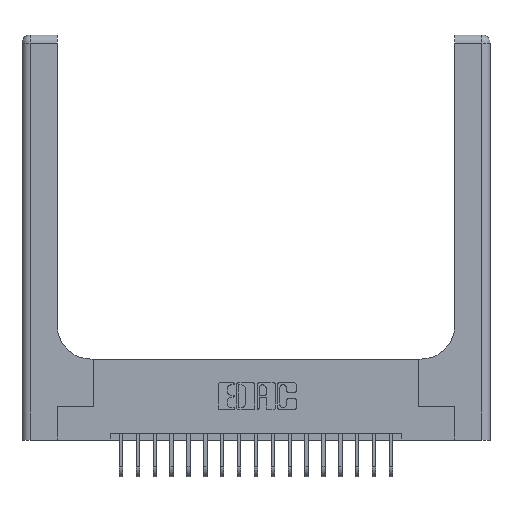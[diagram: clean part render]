
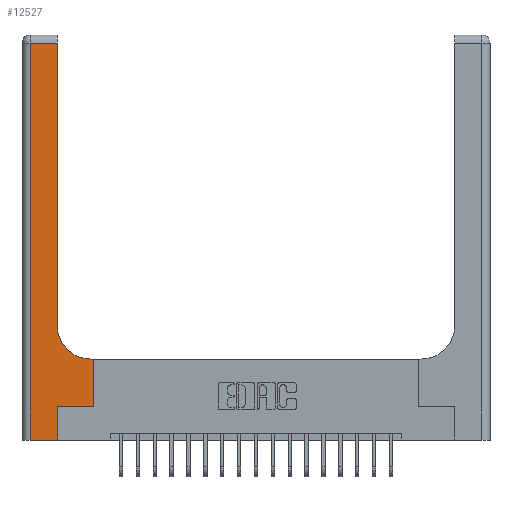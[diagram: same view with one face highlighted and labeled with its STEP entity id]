
A CAD part, top view. The second image highlights one B-rep face of the part: STEP entity #12527.
In plain terms, the highlighted planar face has unit normal (0, 0, 1).
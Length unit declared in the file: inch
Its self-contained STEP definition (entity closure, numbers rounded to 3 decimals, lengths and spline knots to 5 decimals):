
#15 = DIRECTION ( 'NONE',  ( 1., 0., 0. ) ) ;
#594 = VERTEX_POINT ( 'NONE', #11328 ) ;
#892 = CARTESIAN_POINT ( 'NONE',  ( 0.51, 0.85, 0.37 ) ) ;
#1143 = CARTESIAN_POINT ( 'NONE',  ( 0.265, 0., 0.37 ) ) ;
#1306 = VERTEX_POINT ( 'NONE', #5711 ) ;
#1952 = LINE ( 'NONE', #5058, #9387 ) ;
#2213 = LINE ( 'NONE', #4415, #17947 ) ;
#2278 = VECTOR ( 'NONE', #9556, 39.37008 ) ;
#2407 = DIRECTION ( 'NONE',  ( 1., 0., 0. ) ) ;
#2471 = VERTEX_POINT ( 'NONE', #10044 ) ;
#2762 = VERTEX_POINT ( 'NONE', #13661 ) ;
#2944 = VERTEX_POINT ( 'NONE', #16713 ) ;
#3166 = ORIENTED_EDGE ( 'NONE', *, *, #4257, .T. ) ;
#3633 = EDGE_CURVE ( 'NONE', #1306, #2944, #17541, .T. ) ;
#3646 = ORIENTED_EDGE ( 'NONE', *, *, #9079, .T. ) ;
#4257 = EDGE_CURVE ( 'NONE', #17319, #1306, #7355, .T. ) ;
#4364 = CIRCLE ( 'NONE', #14525, 0.25 ) ;
#4415 = CARTESIAN_POINT ( 'NONE',  ( 0.265, 0., 0.37 ) ) ;
#4584 = CARTESIAN_POINT ( 'NONE',  ( 0., 3., 0.37 ) ) ;
#4614 = LINE ( 'NONE', #6154, #12495 ) ;
#5058 = CARTESIAN_POINT ( 'NONE',  ( 0., 2.94, 0.37 ) ) ;
#5375 = FACE_OUTER_BOUND ( 'NONE', #8988, .T. ) ;
#5711 = CARTESIAN_POINT ( 'NONE',  ( 0.528, 0.25, 0.37 ) ) ;
#5756 = ORIENTED_EDGE ( 'NONE', *, *, #7714, .T. ) ;
#5978 = LINE ( 'NONE', #15850, #13363 ) ;
#6038 = DIRECTION ( 'NONE',  ( 0., -1., 0. ) ) ;
#6096 = DIRECTION ( 'NONE',  ( 0., 0., -1. ) ) ;
#6154 = CARTESIAN_POINT ( 'NONE',  ( 0.26, 3., 0.37 ) ) ;
#6441 = VECTOR ( 'NONE', #15, 39.37008 ) ;
#6572 = DIRECTION ( 'NONE',  ( -1., 0., 0. ) ) ;
#6685 = ORIENTED_EDGE ( 'NONE', *, *, #9820, .T. ) ;
#7130 = ORIENTED_EDGE ( 'NONE', *, *, #3633, .T. ) ;
#7355 = LINE ( 'NONE', #17049, #11284 ) ;
#7714 = EDGE_CURVE ( 'NONE', #7873, #9027, #4614, .T. ) ;
#7873 = VERTEX_POINT ( 'NONE', #8068 ) ;
#7988 = EDGE_CURVE ( 'NONE', #2471, #7873, #4364, .T. ) ;
#8068 = CARTESIAN_POINT ( 'NONE',  ( 0.26, 0.85, 0.37 ) ) ;
#8638 = EDGE_CURVE ( 'NONE', #2762, #594, #10373, .T. ) ;
#8982 = AXIS2_PLACEMENT_3D ( 'NONE', #4584, #6096, #16438 ) ;
#8988 = EDGE_LOOP ( 'NONE', ( #5756, #13608, #14086, #17978, #6685, #3166, #7130, #3646, #15479 ) ) ;
#9027 = VERTEX_POINT ( 'NONE', #15782 ) ;
#9079 = EDGE_CURVE ( 'NONE', #2944, #2471, #5978, .T. ) ;
#9387 = VECTOR ( 'NONE', #6572, 39.37008 ) ;
#9556 = DIRECTION ( 'NONE',  ( 0., 1., 0. ) ) ;
#9820 = EDGE_CURVE ( 'NONE', #14719, #17319, #2213, .T. ) ;
#10044 = CARTESIAN_POINT ( 'NONE',  ( 0.51, 0.6, 0.37 ) ) ;
#10077 = EDGE_CURVE ( 'NONE', #9027, #2762, #1952, .T. ) ;
#10373 = LINE ( 'NONE', #17835, #13851 ) ;
#11281 = DIRECTION ( 'NONE',  ( 0., 0., -1. ) ) ;
#11284 = VECTOR ( 'NONE', #14077, 39.37008 ) ;
#11328 = CARTESIAN_POINT ( 'NONE',  ( 0.06, 0., 0.37 ) ) ;
#12495 = VECTOR ( 'NONE', #14993, 39.37008 ) ;
#12527 = ADVANCED_FACE ( 'NONE', ( #5375 ), #13448, .F. ) ;
#13166 = EDGE_CURVE ( 'NONE', #594, #14719, #18150, .T. ) ;
#13274 = DIRECTION ( 'NONE',  ( 0., 1., 0. ) ) ;
#13363 = VECTOR ( 'NONE', #14418, 39.37008 ) ;
#13448 = PLANE ( 'NONE',  #8982 ) ;
#13608 = ORIENTED_EDGE ( 'NONE', *, *, #10077, .T. ) ;
#13661 = CARTESIAN_POINT ( 'NONE',  ( 0.06, 2.94, 0.37 ) ) ;
#13851 = VECTOR ( 'NONE', #6038, 39.37008 ) ;
#13993 = CARTESIAN_POINT ( 'NONE',  ( 0.265, 0.25, 0.37 ) ) ;
#14077 = DIRECTION ( 'NONE',  ( 1., 0., 0. ) ) ;
#14086 = ORIENTED_EDGE ( 'NONE', *, *, #8638, .T. ) ;
#14418 = DIRECTION ( 'NONE',  ( -1., 0., 0. ) ) ;
#14525 = AXIS2_PLACEMENT_3D ( 'NONE', #892, #11281, #2407 ) ;
#14719 = VERTEX_POINT ( 'NONE', #1143 ) ;
#14993 = DIRECTION ( 'NONE',  ( 0., 1., 0. ) ) ;
#15479 = ORIENTED_EDGE ( 'NONE', *, *, #7988, .T. ) ;
#15782 = CARTESIAN_POINT ( 'NONE',  ( 0.26, 2.94, 0.37 ) ) ;
#15850 = CARTESIAN_POINT ( 'NONE',  ( 0.26, 0.6, 0.37 ) ) ;
#16438 = DIRECTION ( 'NONE',  ( -1., 0., 0. ) ) ;
#16713 = CARTESIAN_POINT ( 'NONE',  ( 0.528, 0.6, 0.37 ) ) ;
#17049 = CARTESIAN_POINT ( 'NONE',  ( 0.265, 0.25, 0.37 ) ) ;
#17319 = VERTEX_POINT ( 'NONE', #13993 ) ;
#17541 = LINE ( 'NONE', #18389, #2278 ) ;
#17805 = CARTESIAN_POINT ( 'NONE',  ( 0., 0., 0.37 ) ) ;
#17835 = CARTESIAN_POINT ( 'NONE',  ( 0.06, 3., 0.37 ) ) ;
#17947 = VECTOR ( 'NONE', #13274, 39.37008 ) ;
#17978 = ORIENTED_EDGE ( 'NONE', *, *, #13166, .T. ) ;
#18150 = LINE ( 'NONE', #17805, #6441 ) ;
#18389 = CARTESIAN_POINT ( 'NONE',  ( 0.528, 0.25, 0.37 ) ) ;
